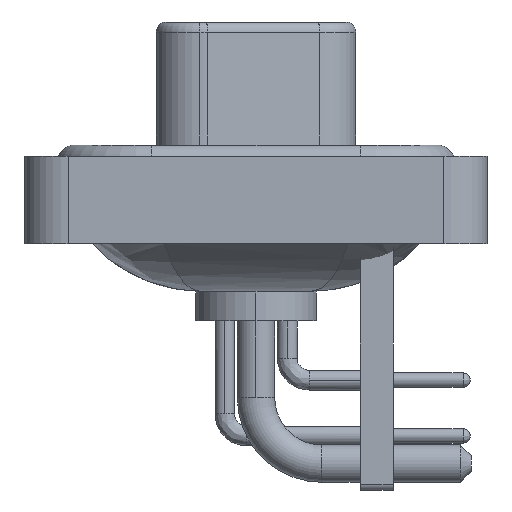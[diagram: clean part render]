
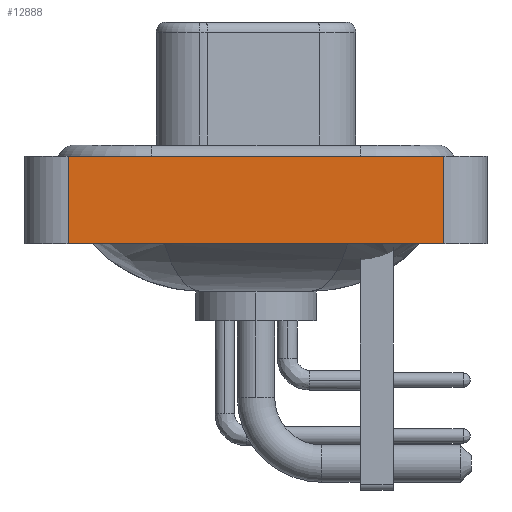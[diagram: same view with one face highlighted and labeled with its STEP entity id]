
A CAD part, left-side view. The second image highlights one B-rep face of the part: STEP entity #12888.
In plain terms, the highlighted planar face has unit normal (-1, 0, 0).
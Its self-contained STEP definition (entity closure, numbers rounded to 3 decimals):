
#840 = ORIENTED_EDGE ( 'NONE', *, *, #16857, .T. ) ;
#2002 = VECTOR ( 'NONE', #7343, 1000. ) ;
#2940 = CARTESIAN_POINT ( 'NONE',  ( -7.35, 8.55, -3.6 ) ) ;
#5180 = CARTESIAN_POINT ( 'NONE',  ( -7.35, -8.55, 0.4 ) ) ;
#5257 = VERTEX_POINT ( 'NONE', #7231 ) ;
#5260 = DIRECTION ( 'NONE',  ( 0., 0., 1. ) ) ;
#5537 = VECTOR ( 'NONE', #21118, 1000. ) ;
#5964 = VERTEX_POINT ( 'NONE', #2940 ) ;
#7231 = CARTESIAN_POINT ( 'NONE',  ( -7.35, 8.55, 0.4 ) ) ;
#7343 = DIRECTION ( 'NONE',  ( 0., -1., 0. ) ) ;
#9540 = ORIENTED_EDGE ( 'NONE', *, *, #18214, .F. ) ;
#10761 = DIRECTION ( 'NONE',  ( 0., 0., 1. ) ) ;
#11483 = CARTESIAN_POINT ( 'NONE',  ( -7.35, -8.55, -3.6 ) ) ;
#11985 = DIRECTION ( 'NONE',  ( -1., 0., 0. ) ) ;
#12397 = PLANE ( 'NONE',  #25215 ) ;
#12794 = CARTESIAN_POINT ( 'NONE',  ( -7.35, -8.55, -3.6 ) ) ;
#12802 = EDGE_LOOP ( 'NONE', ( #840, #9540, #22211, #25910 ) ) ;
#12888 = ADVANCED_FACE ( 'NONE', ( #18416 ), #12397, .T. ) ;
#13606 = EDGE_CURVE ( 'NONE', #5964, #14178, #26005, .T. ) ;
#14178 = VERTEX_POINT ( 'NONE', #25122 ) ;
#14914 = VECTOR ( 'NONE', #10761, 1000. ) ;
#15265 = VECTOR ( 'NONE', #20292, 1000. ) ;
#15720 = VERTEX_POINT ( 'NONE', #17816 ) ;
#16857 = EDGE_CURVE ( 'NONE', #14178, #15720, #16892, .T. ) ;
#16892 = LINE ( 'NONE', #12794, #5537 ) ;
#17336 = CARTESIAN_POINT ( 'NONE',  ( -7.35, 8.55, -3.6 ) ) ;
#17729 = EDGE_CURVE ( 'NONE', #5964, #5257, #21152, .T. ) ;
#17816 = CARTESIAN_POINT ( 'NONE',  ( -7.35, -8.55, 0.4 ) ) ;
#18214 = EDGE_CURVE ( 'NONE', #5257, #15720, #22050, .T. ) ;
#18416 = FACE_OUTER_BOUND ( 'NONE', #12802, .T. ) ;
#20292 = DIRECTION ( 'NONE',  ( 0., -1., 0. ) ) ;
#21118 = DIRECTION ( 'NONE',  ( 0., 0., 1. ) ) ;
#21152 = LINE ( 'NONE', #17336, #14914 ) ;
#22050 = LINE ( 'NONE', #5180, #2002 ) ;
#22177 = CARTESIAN_POINT ( 'NONE',  ( -7.35, -8.55, -3.6 ) ) ;
#22211 = ORIENTED_EDGE ( 'NONE', *, *, #17729, .F. ) ;
#25122 = CARTESIAN_POINT ( 'NONE',  ( -7.35, -8.55, -3.6 ) ) ;
#25215 = AXIS2_PLACEMENT_3D ( 'NONE', #11483, #11985, #5260 ) ;
#25910 = ORIENTED_EDGE ( 'NONE', *, *, #13606, .T. ) ;
#26005 = LINE ( 'NONE', #22177, #15265 ) ;
